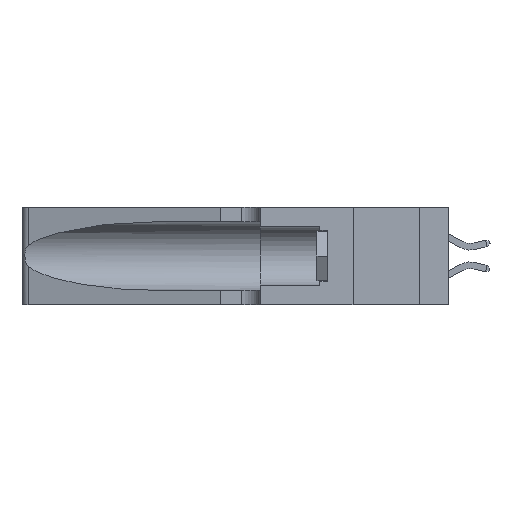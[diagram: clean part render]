
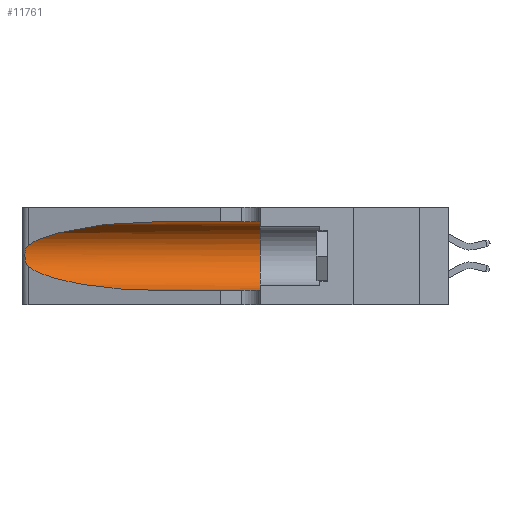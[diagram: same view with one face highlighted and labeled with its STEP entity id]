
A CAD part, left-side view. The second image highlights one B-rep face of the part: STEP entity #11761.
In plain terms, the highlighted cylindrical face has radius 3.308 mm (diameter 6.617 mm), a partial arc.
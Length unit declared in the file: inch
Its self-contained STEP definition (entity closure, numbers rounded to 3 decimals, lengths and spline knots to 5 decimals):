
#322 = EDGE_CURVE ( 'NONE', #2260, #13036, #24126, .T. ) ;
#549 = CARTESIAN_POINT ( 'NONE',  ( 0.25487, 1.22718, 0.22369 ) ) ;
#949 = CARTESIAN_POINT ( 'NONE',  ( 0.25789, 1.23486, 0.15765 ) ) ;
#974 = CARTESIAN_POINT ( 'NONE',  ( 0.18966, 0.96281, 0.05475 ) ) ;
#1115 = DIRECTION ( 'NONE',  ( 0., 0., 1. ) ) ;
#1209 = CARTESIAN_POINT ( 'NONE',  ( 0.1305, 0.35, 0.185 ) ) ;
#1431 = LINE ( 'NONE', #12091, #13825 ) ;
#1977 = DIRECTION ( 'NONE',  ( 0., -1., 0. ) ) ;
#2260 = VERTEX_POINT ( 'NONE', #6219 ) ;
#2344 = EDGE_CURVE ( 'NONE', #23781, #16358, #1431, .T. ) ;
#2502 = DIRECTION ( 'NONE',  ( 0., -1., 0. ) ) ;
#2741 =( BOUNDED_CURVE ( )  B_SPLINE_CURVE ( 3, ( #25547, #7381, #974, #17352 ),
 .UNSPECIFIED., .F., .F. ) 
 B_SPLINE_CURVE_WITH_KNOTS ( ( 4, 4 ),
 ( 3.44316, 4.71239 ),
 .UNSPECIFIED. ) 
 CURVE ( )  GEOMETRIC_REPRESENTATION_ITEM ( )  RATIONAL_B_SPLINE_CURVE ( ( 1., 0.87, 0.87, 1. ) ) 
 REPRESENTATION_ITEM ( '' )  );
#2827 = CARTESIAN_POINT ( 'NONE',  ( 0.26075, 1.23896, 0.19203 ) ) ;
#3015 = CARTESIAN_POINT ( 'NONE',  ( 0.25555, 1.22993, 0.14849 ) ) ;
#3130 = DIRECTION ( 'NONE',  ( 0., -1., 0. ) ) ;
#4233 = ORIENTED_EDGE ( 'NONE', *, *, #4819, .F. ) ;
#4708 = CARTESIAN_POINT ( 'NONE',  ( 0.26017, 1.23833, 0.17102 ) ) ;
#4819 = EDGE_CURVE ( 'NONE', #11522, #21066, #24531, .T. ) ;
#4839 = EDGE_CURVE ( 'NONE', #11522, #2260, #14627, .T. ) ;
#4967 = CARTESIAN_POINT ( 'NONE',  ( 0.25487, 1.22718, 0.22369 ) ) ;
#5258 = DIRECTION ( 'NONE',  ( 0., 0., -1. ) ) ;
#6138 = ORIENTED_EDGE ( 'NONE', *, *, #4839, .T. ) ;
#6219 = CARTESIAN_POINT ( 'NONE',  ( 0.25487, 1.22718, 0.22369 ) ) ;
#7010 = CARTESIAN_POINT ( 'NONE',  ( 0.26075, 1.23896, 0.178 ) ) ;
#7103 = CARTESIAN_POINT ( 'NONE',  ( 0.25787, 1.23484, 0.2124 ) ) ;
#7381 = CARTESIAN_POINT ( 'NONE',  ( 0.2373, 1.15595, 0.08982 ) ) ;
#7422 = CIRCLE ( 'NONE', #17185, 0.13025 ) ;
#7653 = VECTOR ( 'NONE', #2502, 39.37008 ) ;
#7728 = CARTESIAN_POINT ( 'NONE',  ( 0.1305, 0.35, 0.05475 ) ) ;
#8543 = CARTESIAN_POINT ( 'NONE',  ( 0.1305, 0.72297, 0.31525 ) ) ;
#8954 = CARTESIAN_POINT ( 'NONE',  ( 0.25639, 1.23184, 0.21858 ) ) ;
#9391 = DIRECTION ( 'NONE',  ( 0., 1., 0. ) ) ;
#9920 = EDGE_LOOP ( 'NONE', ( #6138, #15178, #25096, #18367, #15780, #4233 ) ) ;
#11522 = VERTEX_POINT ( 'NONE', #12438 ) ;
#11761 = ADVANCED_FACE ( 'NONE', ( #14539 ), #15173, .F. ) ;
#12091 = CARTESIAN_POINT ( 'NONE',  ( 0.1305, 1.61858, 0.05475 ) ) ;
#12122 = CARTESIAN_POINT ( 'NONE',  ( 0.25487, 1.22718, 0.14631 ) ) ;
#12438 = CARTESIAN_POINT ( 'NONE',  ( 0.1305, 0.72297, 0.31525 ) ) ;
#13036 = VERTEX_POINT ( 'NONE', #12122 ) ;
#13122 = CARTESIAN_POINT ( 'NONE',  ( 0.25856, 1.23593, 0.16098 ) ) ;
#13212 = CARTESIAN_POINT ( 'NONE',  ( 0.26018, 1.23835, 0.19895 ) ) ;
#13825 = VECTOR ( 'NONE', #1977, 39.37008 ) ;
#14539 = FACE_OUTER_BOUND ( 'NONE', #9920, .T. ) ;
#14627 =( BOUNDED_CURVE ( )  B_SPLINE_CURVE ( 3, ( #8543, #16818, #22808, #549 ),
 .UNSPECIFIED., .F., .T. ) 
 B_SPLINE_CURVE_WITH_KNOTS ( ( 4, 4 ),
 ( 1.5708, 2.84003 ),
 .UNSPECIFIED. ) 
 CURVE ( )  GEOMETRIC_REPRESENTATION_ITEM ( )  RATIONAL_B_SPLINE_CURVE ( ( 1., 0.87, 0.87, 1. ) ) 
 REPRESENTATION_ITEM ( '' )  );
#15173 = CYLINDRICAL_SURFACE ( 'NONE', #21429, 0.13025 ) ;
#15178 = ORIENTED_EDGE ( 'NONE', *, *, #322, .T. ) ;
#15780 = ORIENTED_EDGE ( 'NONE', *, *, #21973, .F. ) ;
#16358 = VERTEX_POINT ( 'NONE', #7728 ) ;
#16818 = CARTESIAN_POINT ( 'NONE',  ( 0.18966, 0.96281, 0.31525 ) ) ;
#16908 = CARTESIAN_POINT ( 'NONE',  ( 0.1305, 1.61858, 0.31525 ) ) ;
#17185 = AXIS2_PLACEMENT_3D ( 'NONE', #1209, #9391, #1115 ) ;
#17352 = CARTESIAN_POINT ( 'NONE',  ( 0.1305, 0.72297, 0.05475 ) ) ;
#18367 = ORIENTED_EDGE ( 'NONE', *, *, #2344, .T. ) ;
#18859 = CARTESIAN_POINT ( 'NONE',  ( 0.1305, 0.35, 0.31525 ) ) ;
#18930 = CARTESIAN_POINT ( 'NONE',  ( 0.25639, 1.23186, 0.15144 ) ) ;
#19204 = CARTESIAN_POINT ( 'NONE',  ( 0.25854, 1.2359, 0.20912 ) ) ;
#19372 = CARTESIAN_POINT ( 'NONE',  ( 0.1305, 0.72297, 0.05475 ) ) ;
#20714 = EDGE_CURVE ( 'NONE', #13036, #23781, #2741, .T. ) ;
#21066 = VERTEX_POINT ( 'NONE', #18859 ) ;
#21258 = CARTESIAN_POINT ( 'NONE',  ( 0.25487, 1.22718, 0.14631 ) ) ;
#21352 = CARTESIAN_POINT ( 'NONE',  ( 0.25555, 1.22994, 0.2215 ) ) ;
#21371 = CARTESIAN_POINT ( 'NONE',  ( 0.1305, 1.61858, 0.185 ) ) ;
#21429 = AXIS2_PLACEMENT_3D ( 'NONE', #21371, #3130, #5258 ) ;
#21973 = EDGE_CURVE ( 'NONE', #21066, #16358, #7422, .T. ) ;
#22808 = CARTESIAN_POINT ( 'NONE',  ( 0.2373, 1.15595, 0.28018 ) ) ;
#23781 = VERTEX_POINT ( 'NONE', #19372 ) ;
#24126 = B_SPLINE_CURVE_WITH_KNOTS ( 'NONE', 3,
 ( #4967, #21352, #8954, #7103, #19204, #13212, #2827, #7010, #4708, #13122, #949, #18930, #3015, #21258 ),
 .UNSPECIFIED., .F., .F.,
 ( 4, 2, 2, 2, 2, 2, 4 ),
 ( 0., 0.00027, 0.00053, 0.00107, 0.0016, 0.00187, 0.00214 ),
 .UNSPECIFIED. ) ;
#24531 = LINE ( 'NONE', #16908, #7653 ) ;
#25096 = ORIENTED_EDGE ( 'NONE', *, *, #20714, .T. ) ;
#25547 = CARTESIAN_POINT ( 'NONE',  ( 0.25487, 1.22718, 0.14631 ) ) ;
